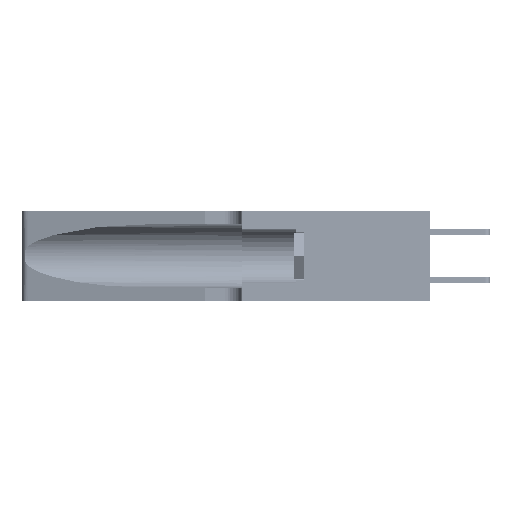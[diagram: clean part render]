
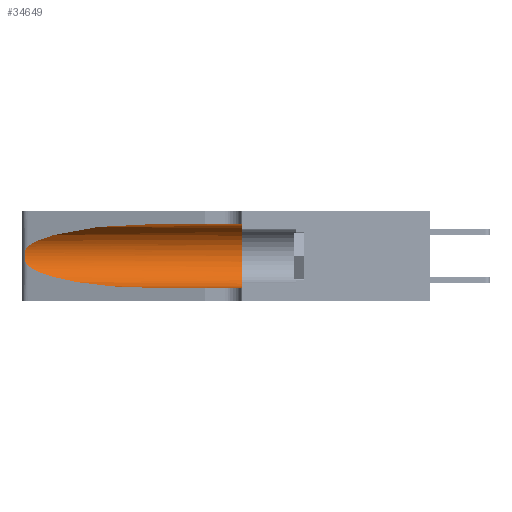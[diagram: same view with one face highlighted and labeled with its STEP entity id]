
A CAD part, left-side view. The second image highlights one B-rep face of the part: STEP entity #34649.
In plain terms, the highlighted cylindrical face has radius 3.308 mm (diameter 6.617 mm), a partial arc.
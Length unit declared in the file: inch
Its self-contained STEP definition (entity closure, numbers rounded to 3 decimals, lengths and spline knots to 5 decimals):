
#1440 = CARTESIAN_POINT ( 'NONE',  ( 0.25487, 1.22718, 0.14631 ) ) ;
#1687 = B_SPLINE_CURVE_WITH_KNOTS ( 'NONE', 3,
 ( #5013, #31320, #8924, #42606, #38525, #9075, #16233, #42274, #16079, #35079, #24042, #19970, #15921, #1440 ),
 .UNSPECIFIED., .F., .F.,
 ( 4, 2, 2, 2, 2, 2, 4 ),
 ( 0., 0.00027, 0.00053, 0.00107, 0.0016, 0.00187, 0.00214 ),
 .UNSPECIFIED. ) ;
#1875 = FACE_OUTER_BOUND ( 'NONE', #6804, .T. ) ;
#4775 = LINE ( 'NONE', #10548, #23377 ) ;
#5013 = CARTESIAN_POINT ( 'NONE',  ( 0.25487, 1.22718, 0.22369 ) ) ;
#5861 = ORIENTED_EDGE ( 'NONE', *, *, #26721, .F. ) ;
#6162 = CARTESIAN_POINT ( 'NONE',  ( 0.25487, 1.22718, 0.14631 ) ) ;
#6277 = EDGE_CURVE ( 'NONE', #34524, #14559, #32572, .T. ) ;
#6804 = EDGE_LOOP ( 'NONE', ( #20039, #7698, #14665, #19466, #5861, #22837 ) ) ;
#7698 = ORIENTED_EDGE ( 'NONE', *, *, #25204, .T. ) ;
#8924 = CARTESIAN_POINT ( 'NONE',  ( 0.25639, 1.23184, 0.21858 ) ) ;
#9075 = CARTESIAN_POINT ( 'NONE',  ( 0.26018, 1.23835, 0.19895 ) ) ;
#10548 = CARTESIAN_POINT ( 'NONE',  ( 0.1305, 1.61858, 0.05475 ) ) ;
#10796 = DIRECTION ( 'NONE',  ( 0., -1., 0. ) ) ;
#10976 = CARTESIAN_POINT ( 'NONE',  ( 0.1305, 0.72297, 0.05475 ) ) ;
#12442 = VERTEX_POINT ( 'NONE', #6162 ) ;
#14559 = VERTEX_POINT ( 'NONE', #33730 ) ;
#14665 = ORIENTED_EDGE ( 'NONE', *, *, #19080, .T. ) ;
#14776 = CARTESIAN_POINT ( 'NONE',  ( 0.25487, 1.22718, 0.14631 ) ) ;
#15441 = EDGE_CURVE ( 'NONE', #34524, #19365, #36262, .T. ) ;
#15768 = VERTEX_POINT ( 'NONE', #10976 ) ;
#15921 = CARTESIAN_POINT ( 'NONE',  ( 0.25555, 1.22993, 0.14849 ) ) ;
#16079 = CARTESIAN_POINT ( 'NONE',  ( 0.26017, 1.23833, 0.17102 ) ) ;
#16233 = CARTESIAN_POINT ( 'NONE',  ( 0.26075, 1.23896, 0.19203 ) ) ;
#17327 = CIRCLE ( 'NONE', #33317, 0.13025 ) ;
#17422 = DIRECTION ( 'NONE',  ( 0., 0., 1. ) ) ;
#17739 = DIRECTION ( 'NONE',  ( 0., -1., 0. ) ) ;
#19080 = EDGE_CURVE ( 'NONE', #12442, #15768, #38954, .T. ) ;
#19365 = VERTEX_POINT ( 'NONE', #42735 ) ;
#19466 = ORIENTED_EDGE ( 'NONE', *, *, #47721, .T. ) ;
#19970 = CARTESIAN_POINT ( 'NONE',  ( 0.25639, 1.23186, 0.15144 ) ) ;
#20039 = ORIENTED_EDGE ( 'NONE', *, *, #15441, .T. ) ;
#20882 = DIRECTION ( 'NONE',  ( 0., -1., 0. ) ) ;
#22837 = ORIENTED_EDGE ( 'NONE', *, *, #6277, .F. ) ;
#23377 = VECTOR ( 'NONE', #17739, 39.37008 ) ;
#23417 = CYLINDRICAL_SURFACE ( 'NONE', #32873, 0.13025 ) ;
#24042 = CARTESIAN_POINT ( 'NONE',  ( 0.25789, 1.23486, 0.15765 ) ) ;
#24506 = VECTOR ( 'NONE', #20882, 39.37008 ) ;
#24924 = DIRECTION ( 'NONE',  ( 0., 1., 0. ) ) ;
#25204 = EDGE_CURVE ( 'NONE', #19365, #12442, #1687, .T. ) ;
#26414 = CARTESIAN_POINT ( 'NONE',  ( 0.1305, 0.35, 0.05475 ) ) ;
#26721 = EDGE_CURVE ( 'NONE', #14559, #39391, #17327, .T. ) ;
#29806 = DIRECTION ( 'NONE',  ( 0., 0., -1. ) ) ;
#31319 = CARTESIAN_POINT ( 'NONE',  ( 0.25487, 1.22718, 0.22369 ) ) ;
#31320 = CARTESIAN_POINT ( 'NONE',  ( 0.25555, 1.22994, 0.2215 ) ) ;
#31651 = CARTESIAN_POINT ( 'NONE',  ( 0.1305, 0.72297, 0.31525 ) ) ;
#32572 = LINE ( 'NONE', #41720, #24506 ) ;
#32873 = AXIS2_PLACEMENT_3D ( 'NONE', #47753, #10796, #29806 ) ;
#33095 = CARTESIAN_POINT ( 'NONE',  ( 0.2373, 1.15595, 0.08982 ) ) ;
#33317 = AXIS2_PLACEMENT_3D ( 'NONE', #39705, #24924, #17422 ) ;
#33730 = CARTESIAN_POINT ( 'NONE',  ( 0.1305, 0.35, 0.31525 ) ) ;
#34524 = VERTEX_POINT ( 'NONE', #47591 ) ;
#34649 = ADVANCED_FACE ( 'NONE', ( #1875 ), #23417, .F. ) ;
#35079 = CARTESIAN_POINT ( 'NONE',  ( 0.25856, 1.23593, 0.16098 ) ) ;
#36262 =( BOUNDED_CURVE ( )  B_SPLINE_CURVE ( 3, ( #31651, #42603, #46188, #31319 ),
 .UNSPECIFIED., .F., .F. ) 
 B_SPLINE_CURVE_WITH_KNOTS ( ( 4, 4 ),
 ( 1.5708, 2.84003 ),
 .UNSPECIFIED. ) 
 CURVE ( )  GEOMETRIC_REPRESENTATION_ITEM ( )  RATIONAL_B_SPLINE_CURVE ( ( 1., 0.87, 0.87, 1. ) ) 
 REPRESENTATION_ITEM ( '' )  );
#38525 = CARTESIAN_POINT ( 'NONE',  ( 0.25854, 1.2359, 0.20912 ) ) ;
#38954 =( BOUNDED_CURVE ( )  B_SPLINE_CURVE ( 3, ( #14776, #33095, #44242, #40798 ),
 .UNSPECIFIED., .F., .T. ) 
 B_SPLINE_CURVE_WITH_KNOTS ( ( 4, 4 ),
 ( 3.44316, 4.71239 ),
 .UNSPECIFIED. ) 
 CURVE ( )  GEOMETRIC_REPRESENTATION_ITEM ( )  RATIONAL_B_SPLINE_CURVE ( ( 1., 0.87, 0.87, 1. ) ) 
 REPRESENTATION_ITEM ( '' )  );
#39391 = VERTEX_POINT ( 'NONE', #26414 ) ;
#39705 = CARTESIAN_POINT ( 'NONE',  ( 0.1305, 0.35, 0.185 ) ) ;
#40798 = CARTESIAN_POINT ( 'NONE',  ( 0.1305, 0.72297, 0.05475 ) ) ;
#41720 = CARTESIAN_POINT ( 'NONE',  ( 0.1305, 1.61858, 0.31525 ) ) ;
#42274 = CARTESIAN_POINT ( 'NONE',  ( 0.26075, 1.23896, 0.178 ) ) ;
#42603 = CARTESIAN_POINT ( 'NONE',  ( 0.18966, 0.96281, 0.31525 ) ) ;
#42606 = CARTESIAN_POINT ( 'NONE',  ( 0.25787, 1.23484, 0.2124 ) ) ;
#42735 = CARTESIAN_POINT ( 'NONE',  ( 0.25487, 1.22718, 0.22369 ) ) ;
#44242 = CARTESIAN_POINT ( 'NONE',  ( 0.18966, 0.96281, 0.05475 ) ) ;
#46188 = CARTESIAN_POINT ( 'NONE',  ( 0.2373, 1.15595, 0.28018 ) ) ;
#47591 = CARTESIAN_POINT ( 'NONE',  ( 0.1305, 0.72297, 0.31525 ) ) ;
#47721 = EDGE_CURVE ( 'NONE', #15768, #39391, #4775, .T. ) ;
#47753 = CARTESIAN_POINT ( 'NONE',  ( 0.1305, 1.61858, 0.185 ) ) ;
